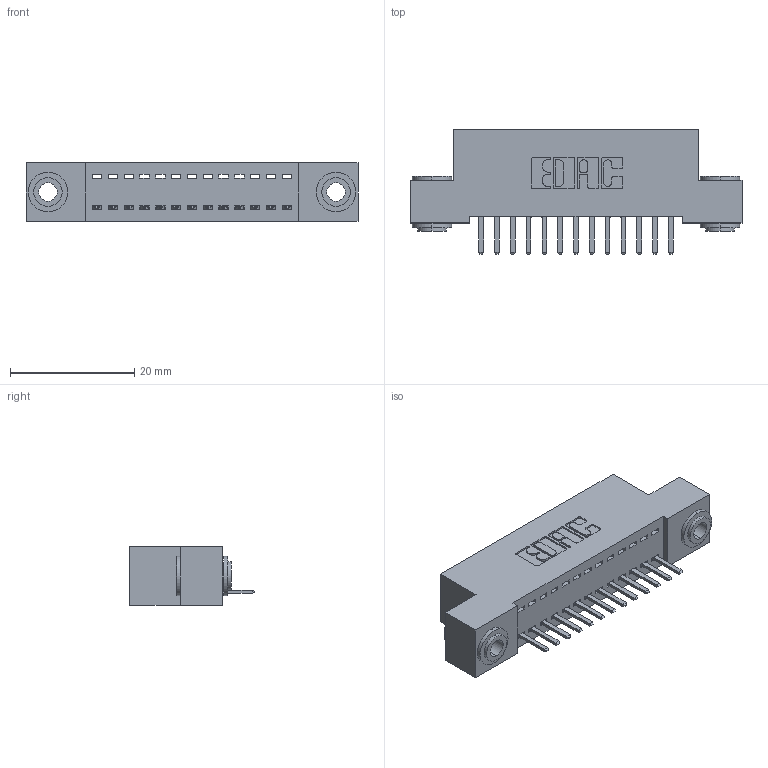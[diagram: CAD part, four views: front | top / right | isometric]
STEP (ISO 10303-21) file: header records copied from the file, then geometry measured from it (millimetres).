
FILE_DESCRIPTION (( 'STEP AP203' ), '1' );
FILE_NAME ('342-013-520-103.STEP', '2018-08-10T16:06:39', ( '' ), ( '' ), 'SwSTEP 2.0', 'SolidWorks 2016', '' );
FILE_SCHEMA (( 'CONFIG_CONTROL_DESIGN' ));
Length unit declared in the file: inch
Products named in the file (4): 345-292-001_345-293-120; 342-250-002_345-250-002-102; 342-013-520-103; 342 Part_.156 TH
Assembly tree (16 placements, depth 2):
  342-013-520-103
    342 Part_.156 TH
    345-292-001_345-293-120  x13
    342-250-002_345-250-002-102  x2
Bounding box: 53.34 x 20.02 x 9.4 mm (x, y, z)
Volume: 4555.5 mm3; surface area: 6254.6 mm2
Topology: 16 solids, 16 shells, 954 faces, 2767 edges, 1806 vertices
Faces by surface type: plane 648, cylinder 298, cone 8
Entity records: 12330 total; most frequent: CARTESIAN_POINT 2120, ORIENTED_EDGE 2050, DIRECTION 1869, EDGE_CURVE 1025, LINE 869, VECTOR 869, VERTEX_POINT 678, AXIS2_PLACEMENT_3D 500
